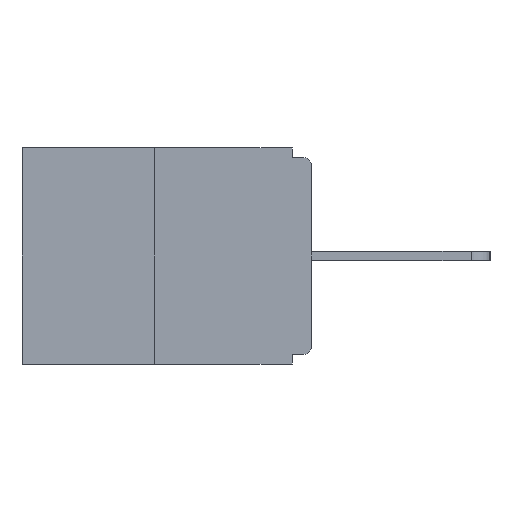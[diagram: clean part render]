
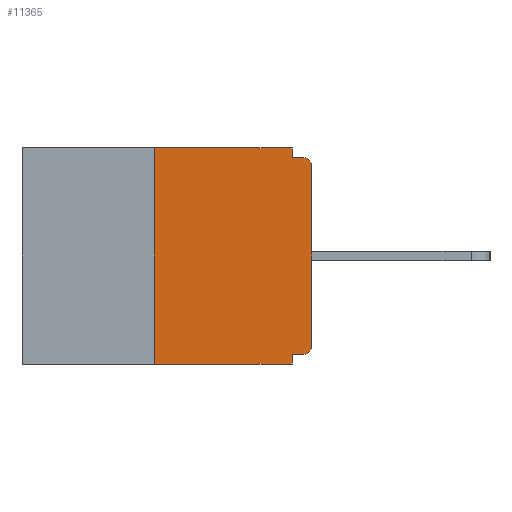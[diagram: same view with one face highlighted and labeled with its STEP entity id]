
A CAD part, left-side view. The second image highlights one B-rep face of the part: STEP entity #11365.
In plain terms, the highlighted planar face has unit normal (-1, 0, 0).
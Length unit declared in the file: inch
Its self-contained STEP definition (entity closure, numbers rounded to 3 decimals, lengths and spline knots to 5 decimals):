
#217 = EDGE_CURVE ( 'NONE', #5907, #1381, #11668, .T. ) ;
#1103 = VECTOR ( 'NONE', #3835, 39.37008 ) ;
#1141 = DIRECTION ( 'NONE',  ( 0., 0., -1. ) ) ;
#1381 = VERTEX_POINT ( 'NONE', #6396 ) ;
#2168 = VECTOR ( 'NONE', #17158, 39.37008 ) ;
#2231 = ORIENTED_EDGE ( 'NONE', *, *, #19642, .F. ) ;
#2350 = CARTESIAN_POINT ( 'NONE',  ( 0., 0.031, -0.328 ) ) ;
#2731 = VECTOR ( 'NONE', #6413, 39.37008 ) ;
#3055 = CARTESIAN_POINT ( 'NONE',  ( 0., 0.46, 0. ) ) ;
#3835 = DIRECTION ( 'NONE',  ( 0., 0., -1. ) ) ;
#4096 = EDGE_CURVE ( 'NONE', #14912, #10798, #17435, .T. ) ;
#4334 = VERTEX_POINT ( 'NONE', #4457 ) ;
#4457 = CARTESIAN_POINT ( 'NONE',  ( 0., 0., -0.313 ) ) ;
#4856 = CARTESIAN_POINT ( 'NONE',  ( 0., 0.015, -0.03 ) ) ;
#5065 = DIRECTION ( 'NONE',  ( 0., 1., 0. ) ) ;
#5326 = DIRECTION ( 'NONE',  ( 0., -1., 0. ) ) ;
#5387 = ORIENTED_EDGE ( 'NONE', *, *, #13234, .T. ) ;
#5407 = LINE ( 'NONE', #6105, #2168 ) ;
#5663 = CARTESIAN_POINT ( 'NONE',  ( 0., 0.25, 0. ) ) ;
#5907 = VERTEX_POINT ( 'NONE', #20441 ) ;
#6035 = CIRCLE ( 'NONE', #16461, 0.015 ) ;
#6105 = CARTESIAN_POINT ( 'NONE',  ( 0., 0.46, 0. ) ) ;
#6130 = VECTOR ( 'NONE', #13424, 39.37008 ) ;
#6242 = DIRECTION ( 'NONE',  ( 0., 0., -1. ) ) ;
#6396 = CARTESIAN_POINT ( 'NONE',  ( 0., 0.031, -0.343 ) ) ;
#6413 = DIRECTION ( 'NONE',  ( 0., -1., 0. ) ) ;
#6445 = DIRECTION ( 'NONE',  ( 0., 0., -1. ) ) ;
#6821 = ORIENTED_EDGE ( 'NONE', *, *, #9310, .T. ) ;
#6880 = ORIENTED_EDGE ( 'NONE', *, *, #17493, .F. ) ;
#6952 = ORIENTED_EDGE ( 'NONE', *, *, #11430, .T. ) ;
#7016 = CARTESIAN_POINT ( 'NONE',  ( 0., 0., -0.03 ) ) ;
#7395 = AXIS2_PLACEMENT_3D ( 'NONE', #8081, #19080, #9654 ) ;
#7587 = ORIENTED_EDGE ( 'NONE', *, *, #217, .T. ) ;
#8081 = CARTESIAN_POINT ( 'NONE',  ( 0., 0.015, -0.313 ) ) ;
#8219 = EDGE_CURVE ( 'NONE', #5907, #15502, #13857, .T. ) ;
#8300 = CARTESIAN_POINT ( 'NONE',  ( 0., 0.031, -0.015 ) ) ;
#8683 = CARTESIAN_POINT ( 'NONE',  ( 0., 0., 0. ) ) ;
#8916 = EDGE_LOOP ( 'NONE', ( #6880, #18502, #7587, #11652, #11428, #5387, #6821, #6952, #2231, #18251 ) ) ;
#9080 = AXIS2_PLACEMENT_3D ( 'NONE', #3055, #15718, #6242 ) ;
#9310 = EDGE_CURVE ( 'NONE', #4334, #14920, #14537, .T. ) ;
#9336 = VECTOR ( 'NONE', #1141, 39.37008 ) ;
#9382 = PLANE ( 'NONE',  #9080 ) ;
#9654 = DIRECTION ( 'NONE',  ( 0., 0., -1. ) ) ;
#9661 = VECTOR ( 'NONE', #16821, 39.37008 ) ;
#10162 = CARTESIAN_POINT ( 'NONE',  ( 0., 0.031, 0. ) ) ;
#10293 = EDGE_CURVE ( 'NONE', #12393, #10524, #15237, .T. ) ;
#10524 = VERTEX_POINT ( 'NONE', #2350 ) ;
#10760 = FACE_OUTER_BOUND ( 'NONE', #8916, .T. ) ;
#10798 = VERTEX_POINT ( 'NONE', #8300 ) ;
#11341 = VECTOR ( 'NONE', #5326, 39.37008 ) ;
#11365 = ADVANCED_FACE ( 'NONE', ( #10760 ), #9382, .F. ) ;
#11428 = ORIENTED_EDGE ( 'NONE', *, *, #10293, .F. ) ;
#11430 = EDGE_CURVE ( 'NONE', #14920, #12268, #6035, .T. ) ;
#11652 = ORIENTED_EDGE ( 'NONE', *, *, #12441, .F. ) ;
#11668 = LINE ( 'NONE', #17678, #2731 ) ;
#11851 = LINE ( 'NONE', #16392, #11341 ) ;
#11943 = CARTESIAN_POINT ( 'NONE',  ( 0., 0.25, 0. ) ) ;
#12050 = VECTOR ( 'NONE', #5065, 39.37008 ) ;
#12268 = VERTEX_POINT ( 'NONE', #16521 ) ;
#12393 = VERTEX_POINT ( 'NONE', #15266 ) ;
#12441 = EDGE_CURVE ( 'NONE', #10524, #1381, #17711, .T. ) ;
#13234 = EDGE_CURVE ( 'NONE', #12393, #4334, #15454, .T. ) ;
#13424 = DIRECTION ( 'NONE',  ( 0., 0., 1. ) ) ;
#13822 = CARTESIAN_POINT ( 'NONE',  ( 0., 0.031, -0.343 ) ) ;
#13857 = LINE ( 'NONE', #11943, #9661 ) ;
#14537 = LINE ( 'NONE', #8683, #6130 ) ;
#14538 = CARTESIAN_POINT ( 'NONE',  ( 0., 0., -0.328 ) ) ;
#14912 = VERTEX_POINT ( 'NONE', #19618 ) ;
#14920 = VERTEX_POINT ( 'NONE', #7016 ) ;
#15237 = LINE ( 'NONE', #14538, #12050 ) ;
#15266 = CARTESIAN_POINT ( 'NONE',  ( 0., 0.015, -0.328 ) ) ;
#15454 = CIRCLE ( 'NONE', #7395, 0.015 ) ;
#15502 = VERTEX_POINT ( 'NONE', #5663 ) ;
#15718 = DIRECTION ( 'NONE',  ( 1., 0., 0. ) ) ;
#15904 = DIRECTION ( 'NONE',  ( -1., 0., 0. ) ) ;
#16392 = CARTESIAN_POINT ( 'NONE',  ( 0., 0., -0.015 ) ) ;
#16461 = AXIS2_PLACEMENT_3D ( 'NONE', #4856, #15904, #6445 ) ;
#16521 = CARTESIAN_POINT ( 'NONE',  ( 0., 0.015, -0.015 ) ) ;
#16821 = DIRECTION ( 'NONE',  ( 0., 0., 1. ) ) ;
#17158 = DIRECTION ( 'NONE',  ( 0., -1., 0. ) ) ;
#17435 = LINE ( 'NONE', #10162, #1103 ) ;
#17493 = EDGE_CURVE ( 'NONE', #15502, #14912, #5407, .T. ) ;
#17678 = CARTESIAN_POINT ( 'NONE',  ( 0., 0.46, -0.343 ) ) ;
#17711 = LINE ( 'NONE', #13822, #9336 ) ;
#18251 = ORIENTED_EDGE ( 'NONE', *, *, #4096, .F. ) ;
#18502 = ORIENTED_EDGE ( 'NONE', *, *, #8219, .F. ) ;
#19080 = DIRECTION ( 'NONE',  ( -1., 0., 0. ) ) ;
#19618 = CARTESIAN_POINT ( 'NONE',  ( 0., 0.031, 0. ) ) ;
#19642 = EDGE_CURVE ( 'NONE', #10798, #12268, #11851, .T. ) ;
#20441 = CARTESIAN_POINT ( 'NONE',  ( 0., 0.25, -0.343 ) ) ;
